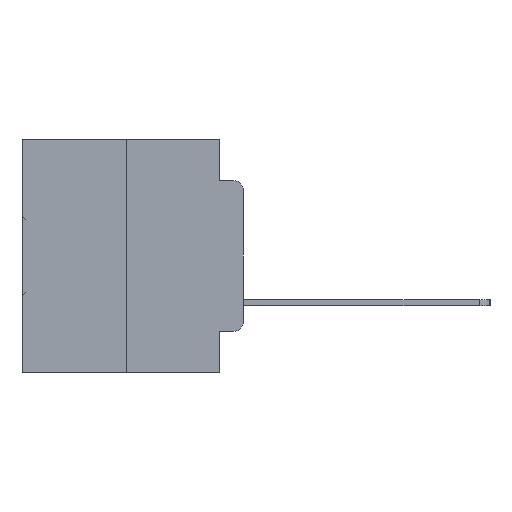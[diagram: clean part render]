
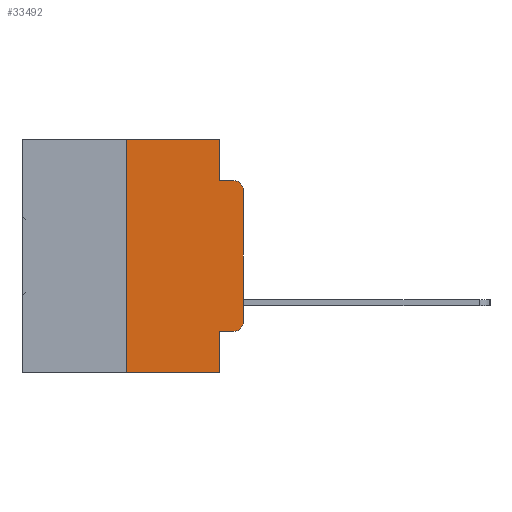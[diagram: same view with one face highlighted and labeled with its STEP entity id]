
A CAD part, left-side view. The second image highlights one B-rep face of the part: STEP entity #33492.
In plain terms, the highlighted planar face has unit normal (-1, 0, 0).
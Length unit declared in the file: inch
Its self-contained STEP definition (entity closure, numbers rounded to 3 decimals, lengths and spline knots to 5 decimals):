
#437 = CARTESIAN_POINT ( 'NONE',  ( 0., 0.473, -0.5 ) ) ;
#707 = VECTOR ( 'NONE', #11208, 39.37008 ) ;
#1155 = LINE ( 'NONE', #9666, #27204 ) ;
#1492 = DIRECTION ( 'NONE',  ( 0., 0., -1. ) ) ;
#1794 = LINE ( 'NONE', #29133, #15979 ) ;
#2001 = EDGE_CURVE ( 'NONE', #22800, #6320, #17460, .T. ) ;
#2017 = CARTESIAN_POINT ( 'NONE',  ( 0., 0.051, -0.0885 ) ) ;
#2946 = EDGE_CURVE ( 'NONE', #11733, #28382, #10458, .T. ) ;
#3133 = DIRECTION ( 'NONE',  ( 0., -1., 0. ) ) ;
#4387 = AXIS2_PLACEMENT_3D ( 'NONE', #11024, #28860, #13687 ) ;
#4648 = CARTESIAN_POINT ( 'NONE',  ( 0., 0.25, -0.5 ) ) ;
#6147 = EDGE_CURVE ( 'NONE', #25022, #11733, #14196, .T. ) ;
#6320 = VERTEX_POINT ( 'NONE', #2017 ) ;
#6665 = VECTOR ( 'NONE', #3133, 39.37008 ) ;
#6826 = EDGE_CURVE ( 'NONE', #30993, #25537, #1155, .T. ) ;
#6829 = ORIENTED_EDGE ( 'NONE', *, *, #20008, .F. ) ;
#6918 = DIRECTION ( 'NONE',  ( 0., 0., -1. ) ) ;
#7607 = VERTEX_POINT ( 'NONE', #25539 ) ;
#8525 = FACE_OUTER_BOUND ( 'NONE', #11795, .T. ) ;
#8555 = CARTESIAN_POINT ( 'NONE',  ( 0., 0.473, 0. ) ) ;
#9321 = CARTESIAN_POINT ( 'NONE',  ( 0., 0., -0.3915 ) ) ;
#9666 = CARTESIAN_POINT ( 'NONE',  ( 0., 0.051, 0. ) ) ;
#9719 = VERTEX_POINT ( 'NONE', #28568 ) ;
#10458 = LINE ( 'NONE', #28613, #24116 ) ;
#10519 = CARTESIAN_POINT ( 'NONE',  ( 0., 0.02, -0.4115 ) ) ;
#10529 = VECTOR ( 'NONE', #22631, 39.37008 ) ;
#11010 = EDGE_CURVE ( 'NONE', #24912, #9719, #30822, .T. ) ;
#11024 = CARTESIAN_POINT ( 'NONE',  ( 0., 0.02, -0.1085 ) ) ;
#11041 = ORIENTED_EDGE ( 'NONE', *, *, #6147, .T. ) ;
#11208 = DIRECTION ( 'NONE',  ( 0., -1., 0. ) ) ;
#11657 = CARTESIAN_POINT ( 'NONE',  ( 0., 0.25, 0. ) ) ;
#11733 = VERTEX_POINT ( 'NONE', #9321 ) ;
#11795 = EDGE_LOOP ( 'NONE', ( #32523, #32189, #33322, #27395, #6829, #28203, #23104, #23889, #14772, #11041 ) ) ;
#11797 = CARTESIAN_POINT ( 'NONE',  ( 0., 0.051, -0.0885 ) ) ;
#12204 = PLANE ( 'NONE',  #23272 ) ;
#13687 = DIRECTION ( 'NONE',  ( 0., 0., -1. ) ) ;
#13968 = DIRECTION ( 'NONE',  ( 0., -1., 0. ) ) ;
#14196 = CIRCLE ( 'NONE', #29451, 0.02 ) ;
#14749 = DIRECTION ( 'NONE',  ( -1., 0., 0. ) ) ;
#14772 = ORIENTED_EDGE ( 'NONE', *, *, #25232, .T. ) ;
#14827 = CARTESIAN_POINT ( 'NONE',  ( 0., 0.473, 0. ) ) ;
#15845 = EDGE_CURVE ( 'NONE', #6320, #7607, #19476, .T. ) ;
#15853 = VECTOR ( 'NONE', #21976, 39.37008 ) ;
#15979 = VECTOR ( 'NONE', #13968, 39.37008 ) ;
#17415 = DIRECTION ( 'NONE',  ( 1., 0., 0. ) ) ;
#17460 = LINE ( 'NONE', #32639, #10529 ) ;
#17876 = CARTESIAN_POINT ( 'NONE',  ( 0., 0.051, -0.5 ) ) ;
#17904 = VECTOR ( 'NONE', #22104, 39.37008 ) ;
#19476 = LINE ( 'NONE', #11797, #17904 ) ;
#20008 = EDGE_CURVE ( 'NONE', #9719, #22800, #21677, .T. ) ;
#20924 = CIRCLE ( 'NONE', #4387, 0.02 ) ;
#21025 = DIRECTION ( 'NONE',  ( 0., 0., 1. ) ) ;
#21677 = LINE ( 'NONE', #8555, #707 ) ;
#21976 = DIRECTION ( 'NONE',  ( 0., 0., 1. ) ) ;
#22104 = DIRECTION ( 'NONE',  ( 0., -1., 0. ) ) ;
#22631 = DIRECTION ( 'NONE',  ( 0., 0., -1. ) ) ;
#22800 = VERTEX_POINT ( 'NONE', #32227 ) ;
#23104 = ORIENTED_EDGE ( 'NONE', *, *, #28213, .T. ) ;
#23272 = AXIS2_PLACEMENT_3D ( 'NONE', #14827, #17415, #1492 ) ;
#23889 = ORIENTED_EDGE ( 'NONE', *, *, #6826, .F. ) ;
#24116 = VECTOR ( 'NONE', #21025, 39.37008 ) ;
#24633 = CARTESIAN_POINT ( 'NONE',  ( 0., 0.051, -0.4115 ) ) ;
#24912 = VERTEX_POINT ( 'NONE', #4648 ) ;
#25022 = VERTEX_POINT ( 'NONE', #10519 ) ;
#25232 = EDGE_CURVE ( 'NONE', #30993, #25022, #1794, .T. ) ;
#25537 = VERTEX_POINT ( 'NONE', #17876 ) ;
#25539 = CARTESIAN_POINT ( 'NONE',  ( 0., 0.02, -0.0885 ) ) ;
#27204 = VECTOR ( 'NONE', #6918, 39.37008 ) ;
#27236 = LINE ( 'NONE', #437, #6665 ) ;
#27395 = ORIENTED_EDGE ( 'NONE', *, *, #2001, .F. ) ;
#28203 = ORIENTED_EDGE ( 'NONE', *, *, #11010, .F. ) ;
#28213 = EDGE_CURVE ( 'NONE', #24912, #25537, #27236, .T. ) ;
#28382 = VERTEX_POINT ( 'NONE', #29692 ) ;
#28568 = CARTESIAN_POINT ( 'NONE',  ( 0., 0.25, 0. ) ) ;
#28613 = CARTESIAN_POINT ( 'NONE',  ( 0., 0., 0. ) ) ;
#28860 = DIRECTION ( 'NONE',  ( -1., 0., 0. ) ) ;
#29133 = CARTESIAN_POINT ( 'NONE',  ( 0., 0.051, -0.4115 ) ) ;
#29416 = EDGE_CURVE ( 'NONE', #28382, #7607, #20924, .T. ) ;
#29451 = AXIS2_PLACEMENT_3D ( 'NONE', #29888, #14749, #32428 ) ;
#29692 = CARTESIAN_POINT ( 'NONE',  ( 0., 0., -0.1085 ) ) ;
#29888 = CARTESIAN_POINT ( 'NONE',  ( 0., 0.02, -0.3915 ) ) ;
#30822 = LINE ( 'NONE', #11657, #15853 ) ;
#30993 = VERTEX_POINT ( 'NONE', #24633 ) ;
#32189 = ORIENTED_EDGE ( 'NONE', *, *, #29416, .T. ) ;
#32227 = CARTESIAN_POINT ( 'NONE',  ( 0., 0.051, 0. ) ) ;
#32428 = DIRECTION ( 'NONE',  ( 0., 0., -1. ) ) ;
#32523 = ORIENTED_EDGE ( 'NONE', *, *, #2946, .T. ) ;
#32639 = CARTESIAN_POINT ( 'NONE',  ( 0., 0.051, 0. ) ) ;
#33322 = ORIENTED_EDGE ( 'NONE', *, *, #15845, .F. ) ;
#33492 = ADVANCED_FACE ( 'NONE', ( #8525 ), #12204, .F. ) ;
